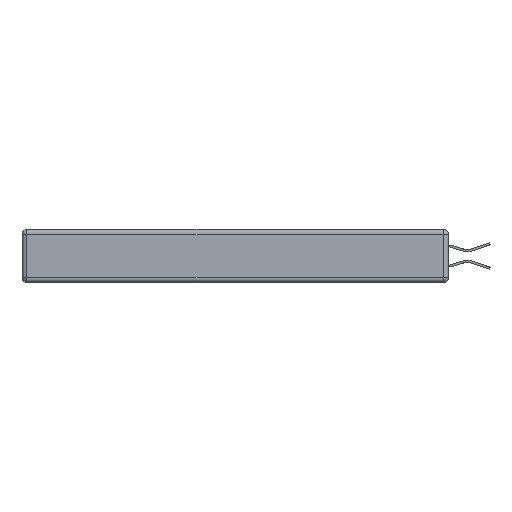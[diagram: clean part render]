
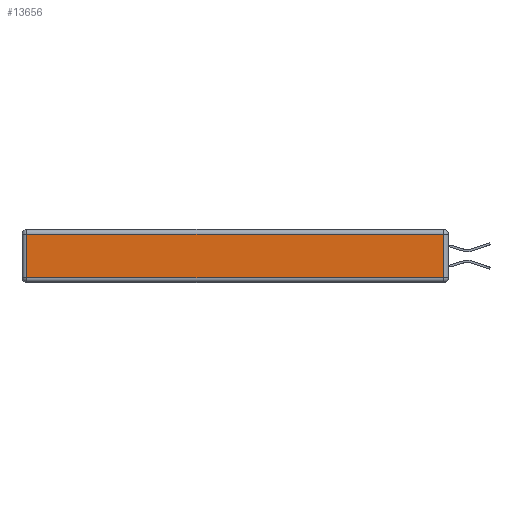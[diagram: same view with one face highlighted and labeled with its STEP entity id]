
A CAD part, left-side view. The second image highlights one B-rep face of the part: STEP entity #13656.
In plain terms, the highlighted planar face has unit normal (-1, 0, 0).
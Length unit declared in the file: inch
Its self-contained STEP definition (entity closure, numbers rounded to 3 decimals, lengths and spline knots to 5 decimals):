
#246 = VECTOR ( 'NONE', #1678, 39.37008 ) ;
#906 = CARTESIAN_POINT ( 'NONE',  ( 0., 0., -0.343 ) ) ;
#1299 = VECTOR ( 'NONE', #11884, 39.37008 ) ;
#1366 = VERTEX_POINT ( 'NONE', #13530 ) ;
#1678 = DIRECTION ( 'NONE',  ( 0., -1., 0. ) ) ;
#1975 = CARTESIAN_POINT ( 'NONE',  ( 0., 2.72, -0.313 ) ) ;
#2158 = ORIENTED_EDGE ( 'NONE', *, *, #5086, .T. ) ;
#2397 = CARTESIAN_POINT ( 'NONE',  ( 0., 2.72, -0.343 ) ) ;
#2914 = CARTESIAN_POINT ( 'NONE',  ( 0., 0., -0.313 ) ) ;
#3148 = VERTEX_POINT ( 'NONE', #1975 ) ;
#3490 = VERTEX_POINT ( 'NONE', #4765 ) ;
#4390 = FACE_OUTER_BOUND ( 'NONE', #5887, .T. ) ;
#4563 = LINE ( 'NONE', #9651, #1299 ) ;
#4765 = CARTESIAN_POINT ( 'NONE',  ( 0., 2.72, -0.03 ) ) ;
#5086 = EDGE_CURVE ( 'NONE', #3490, #3148, #13884, .T. ) ;
#5887 = EDGE_LOOP ( 'NONE', ( #8277, #6303, #11611, #2158 ) ) ;
#6303 = ORIENTED_EDGE ( 'NONE', *, *, #7253, .T. ) ;
#6619 = VECTOR ( 'NONE', #9717, 39.37008 ) ;
#6854 = DIRECTION ( 'NONE',  ( 0., 0., -1. ) ) ;
#7253 = EDGE_CURVE ( 'NONE', #10724, #1366, #10940, .T. ) ;
#8277 = ORIENTED_EDGE ( 'NONE', *, *, #9538, .T. ) ;
#8590 = CARTESIAN_POINT ( 'NONE',  ( 0., 0.03, -0.313 ) ) ;
#9538 = EDGE_CURVE ( 'NONE', #3148, #10724, #12519, .T. ) ;
#9651 = CARTESIAN_POINT ( 'NONE',  ( 0., 2.75, -0.03 ) ) ;
#9687 = DIRECTION ( 'NONE',  ( -1., 0., 0. ) ) ;
#9717 = DIRECTION ( 'NONE',  ( 0., 0., 1. ) ) ;
#10673 = DIRECTION ( 'NONE',  ( 0., 0., 1. ) ) ;
#10724 = VERTEX_POINT ( 'NONE', #8590 ) ;
#10940 = LINE ( 'NONE', #14095, #6619 ) ;
#11611 = ORIENTED_EDGE ( 'NONE', *, *, #13209, .T. ) ;
#11884 = DIRECTION ( 'NONE',  ( 0., 1., 0. ) ) ;
#12519 = LINE ( 'NONE', #2914, #246 ) ;
#12566 = AXIS2_PLACEMENT_3D ( 'NONE', #906, #9687, #10673 ) ;
#13209 = EDGE_CURVE ( 'NONE', #1366, #3490, #4563, .T. ) ;
#13365 = VECTOR ( 'NONE', #6854, 39.37008 ) ;
#13530 = CARTESIAN_POINT ( 'NONE',  ( 0., 0.03, -0.03 ) ) ;
#13656 = ADVANCED_FACE ( 'NONE', ( #4390 ), #14021, .T. ) ;
#13884 = LINE ( 'NONE', #2397, #13365 ) ;
#14021 = PLANE ( 'NONE',  #12566 ) ;
#14095 = CARTESIAN_POINT ( 'NONE',  ( 0., 0.03, -0.343 ) ) ;
